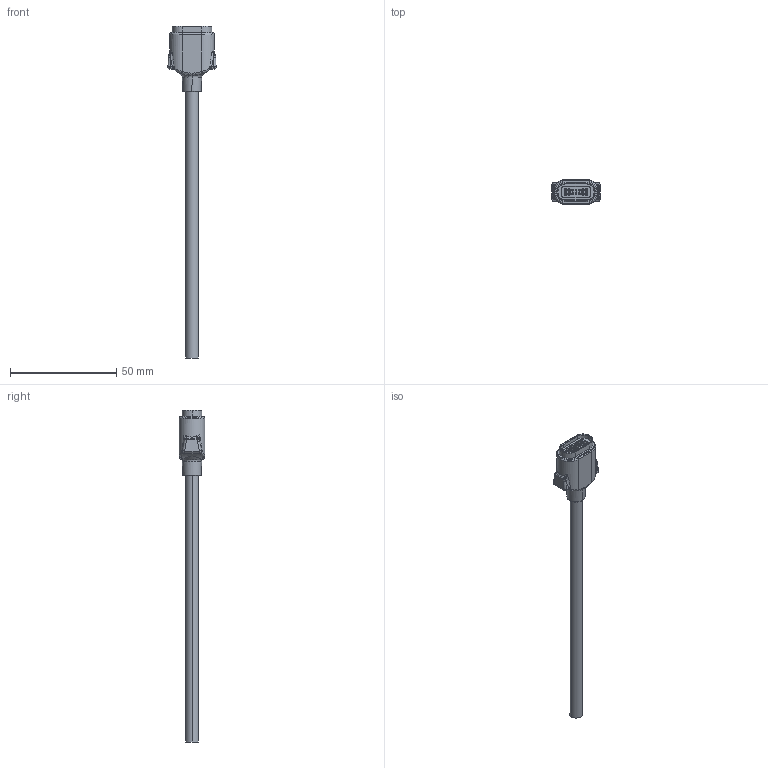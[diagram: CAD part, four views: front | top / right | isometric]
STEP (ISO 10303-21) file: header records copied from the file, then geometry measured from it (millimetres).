
FILE_DESCRIPTION (( 'STEP AP214' ), '1' );
FILE_NAME ('687A14140601100.STEP', '2023-05-02T14:47:24', ( '' ), ( '' ), 'SwSTEP 2.0', 'SolidWorks 2020', '' );
FILE_SCHEMA (( 'AUTOMOTIVE_DESIGN' ));
Length unit declared in the file: millimetre
Products named in the file (1): 687A14140601100
Bounding box: 22.64 x 12 x 156 mm (x, y, z)
Volume: 8603 mm3; surface area: 4331 mm2
Topology: 1 solids, 1 shells, 258 faces, 623 edges, 364 vertices
Faces by surface type: cylinder 96, bspline 54, plane 49, sphere 36, torus 13, cone 10
Entity records: 11024 total; most frequent: CARTESIAN_POINT 4504, DIRECTION 1152, ORIENTED_EDGE 1110, EDGE_CURVE 555, AXIS2_PLACEMENT_3D 492, VERTEX_POINT 332, EDGE_LOOP 291, CIRCLE 287
